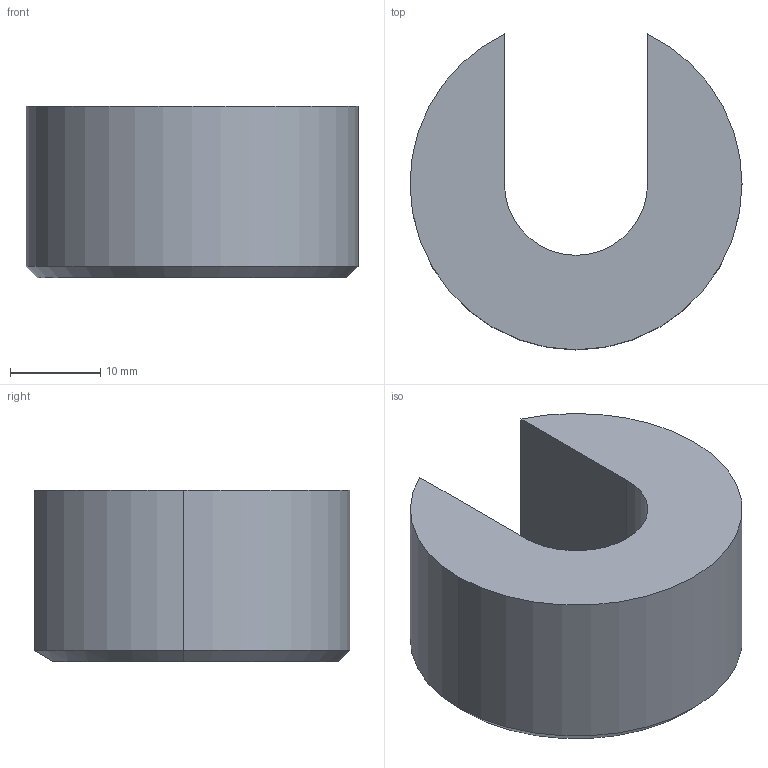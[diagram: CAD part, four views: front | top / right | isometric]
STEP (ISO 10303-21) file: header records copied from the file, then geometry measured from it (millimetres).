
FILE_DESCRIPTION (( 'STEP AP203' ), '1' );
FILE_NAME ('AF-RUGER1022NT-NTMCD-PRT-004-STEP.STEP', '2020-08-27T22:59:45', ( '' ), ( '' ), 'SwSTEP 2.0', 'SolidWorks 2018', '' );
FILE_SCHEMA (( 'CONFIG_CONTROL_DESIGN' ));
Length unit declared in the file: inch
Products named in the file (1): AF-RUGER1022NT-NTMCD-PRT-004-STEP
Bounding box: 36.83 x 35.03 x 19.05 mm (x, y, z)
Volume: 12894.2 mm3; surface area: 4246.3 mm2
Topology: 1 solids, 1 shells, 14 faces, 30 edges, 18 vertices
Faces by surface type: plane 6, cone 4, cylinder 4
Entity records: 459 total; most frequent: DIRECTION 70, CARTESIAN_POINT 69, ORIENTED_EDGE 60, EDGE_CURVE 30, AXIS2_PLACEMENT_3D 27, VERTEX_POINT 18, VECTOR 16, LINE 16
